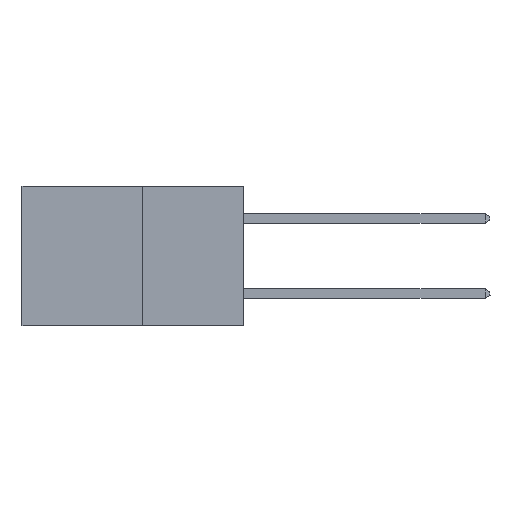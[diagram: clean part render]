
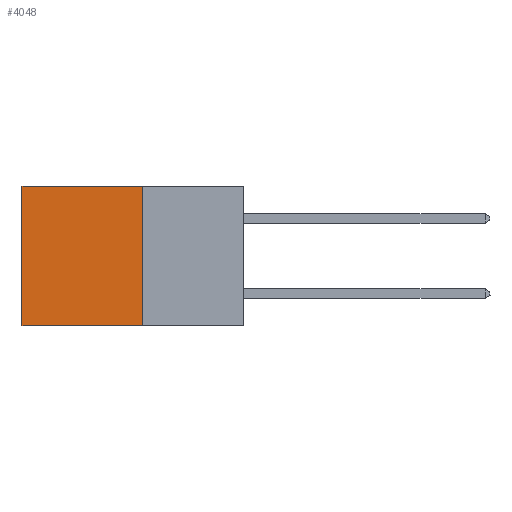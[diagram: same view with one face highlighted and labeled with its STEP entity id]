
A CAD part, left-side view. The second image highlights one B-rep face of the part: STEP entity #4048.
In plain terms, the highlighted planar face has unit normal (-1, 0, 0).
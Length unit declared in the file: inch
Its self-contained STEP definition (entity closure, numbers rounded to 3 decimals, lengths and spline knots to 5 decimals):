
#400 = LINE ( 'NONE', #4169, #5042 ) ;
#518 = EDGE_CURVE ( 'NONE', #2817, #2995, #400, .T. ) ;
#912 = LINE ( 'NONE', #2296, #7574 ) ;
#934 = CARTESIAN_POINT ( 'NONE',  ( 0.277, 0.27, 0. ) ) ;
#1878 = CARTESIAN_POINT ( 'NONE',  ( 0.277, 0.59, 0. ) ) ;
#1946 = EDGE_CURVE ( 'NONE', #11069, #2817, #2488, .T. ) ;
#1996 = DIRECTION ( 'NONE',  ( 0., 1., 0. ) ) ;
#2003 = EDGE_LOOP ( 'NONE', ( #3141, #3558, #3712, #3992 ) ) ;
#2258 = EDGE_CURVE ( 'NONE', #11069, #7623, #912, .T. ) ;
#2296 = CARTESIAN_POINT ( 'NONE',  ( 0.277, 0.27, 0. ) ) ;
#2488 = LINE ( 'NONE', #6635, #3823 ) ;
#2627 = CARTESIAN_POINT ( 'NONE',  ( 0.277, 0.59, -0.37 ) ) ;
#2817 = VERTEX_POINT ( 'NONE', #4800 ) ;
#2995 = VERTEX_POINT ( 'NONE', #2627 ) ;
#3141 = ORIENTED_EDGE ( 'NONE', *, *, #3527, .T. ) ;
#3527 = EDGE_CURVE ( 'NONE', #7623, #2995, #8746, .T. ) ;
#3558 = ORIENTED_EDGE ( 'NONE', *, *, #518, .F. ) ;
#3712 = ORIENTED_EDGE ( 'NONE', *, *, #1946, .F. ) ;
#3823 = VECTOR ( 'NONE', #4704, 39.37008 ) ;
#3992 = ORIENTED_EDGE ( 'NONE', *, *, #2258, .T. ) ;
#3996 = AXIS2_PLACEMENT_3D ( 'NONE', #4603, #4591, #4560 ) ;
#4048 = ADVANCED_FACE ( 'NONE', ( #4482 ), #4969, .F. ) ;
#4089 = VECTOR ( 'NONE', #9272, 39.37008 ) ;
#4169 = CARTESIAN_POINT ( 'NONE',  ( 0.277, 0.27, -0.37 ) ) ;
#4482 = FACE_OUTER_BOUND ( 'NONE', #2003, .T. ) ;
#4560 = DIRECTION ( 'NONE',  ( 0., 0., -1. ) ) ;
#4591 = DIRECTION ( 'NONE',  ( 1., 0., 0. ) ) ;
#4603 = CARTESIAN_POINT ( 'NONE',  ( 0.277, 0.27, -0.37 ) ) ;
#4704 = DIRECTION ( 'NONE',  ( 0., 0., -1. ) ) ;
#4800 = CARTESIAN_POINT ( 'NONE',  ( 0.277, 0.27, -0.37 ) ) ;
#4969 = PLANE ( 'NONE',  #3996 ) ;
#5042 = VECTOR ( 'NONE', #1996, 39.37008 ) ;
#6635 = CARTESIAN_POINT ( 'NONE',  ( 0.277, 0.27, -0.37 ) ) ;
#7574 = VECTOR ( 'NONE', #10578, 39.37008 ) ;
#7623 = VERTEX_POINT ( 'NONE', #1878 ) ;
#8746 = LINE ( 'NONE', #9302, #4089 ) ;
#9272 = DIRECTION ( 'NONE',  ( 0., 0., -1. ) ) ;
#9302 = CARTESIAN_POINT ( 'NONE',  ( 0.277, 0.59, -0.37 ) ) ;
#10578 = DIRECTION ( 'NONE',  ( 0., 1., 0. ) ) ;
#11069 = VERTEX_POINT ( 'NONE', #934 ) ;
